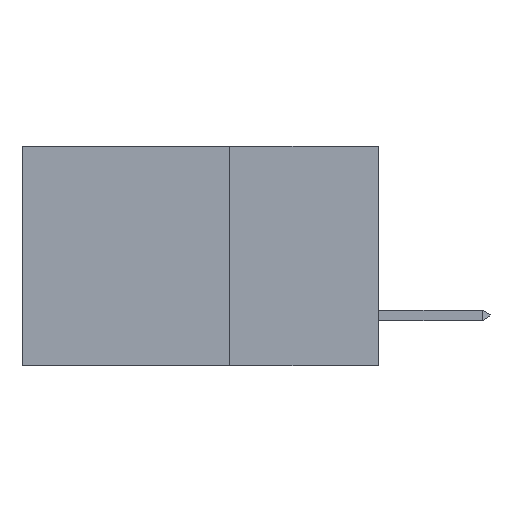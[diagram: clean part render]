
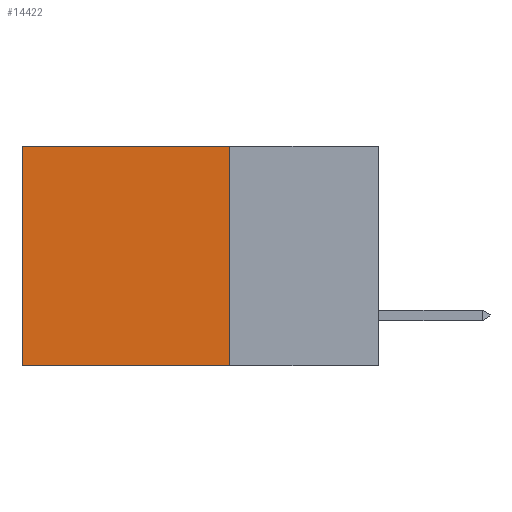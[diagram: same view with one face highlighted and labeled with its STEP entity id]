
A CAD part, left-side view. The second image highlights one B-rep face of the part: STEP entity #14422.
In plain terms, the highlighted planar face has unit normal (-1, 0, 0).
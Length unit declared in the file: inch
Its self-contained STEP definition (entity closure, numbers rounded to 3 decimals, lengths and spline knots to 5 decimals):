
#515 = CARTESIAN_POINT ( 'NONE',  ( 0.298, 0.25, 0. ) ) ;
#547 = CARTESIAN_POINT ( 'NONE',  ( 0.298, 0.6, 0. ) ) ;
#1889 = DIRECTION ( 'NONE',  ( 1., 0., 0. ) ) ;
#2542 = ORIENTED_EDGE ( 'NONE', *, *, #6276, .T. ) ;
#2660 = LINE ( 'NONE', #14740, #15370 ) ;
#3211 = EDGE_CURVE ( 'NONE', #7305, #8714, #5840, .T. ) ;
#3430 = EDGE_LOOP ( 'NONE', ( #2542, #12902, #21877, #7335 ) ) ;
#3825 = CARTESIAN_POINT ( 'NONE',  ( 0.298, 0.25, 0. ) ) ;
#4298 = LINE ( 'NONE', #515, #23408 ) ;
#5840 = LINE ( 'NONE', #8476, #15121 ) ;
#6066 = VERTEX_POINT ( 'NONE', #10850 ) ;
#6276 = EDGE_CURVE ( 'NONE', #6066, #8714, #20544, .T. ) ;
#6742 = EDGE_CURVE ( 'NONE', #23928, #6066, #4298, .T. ) ;
#6780 = DIRECTION ( 'NONE',  ( 0., 1., 0. ) ) ;
#7305 = VERTEX_POINT ( 'NONE', #9884 ) ;
#7335 = ORIENTED_EDGE ( 'NONE', *, *, #6742, .T. ) ;
#8476 = CARTESIAN_POINT ( 'NONE',  ( 0.298, 0.25, -0.37 ) ) ;
#8644 = VECTOR ( 'NONE', #15340, 39.37008 ) ;
#8714 = VERTEX_POINT ( 'NONE', #11927 ) ;
#9884 = CARTESIAN_POINT ( 'NONE',  ( 0.298, 0.25, -0.37 ) ) ;
#10850 = CARTESIAN_POINT ( 'NONE',  ( 0.298, 0.6, 0. ) ) ;
#11927 = CARTESIAN_POINT ( 'NONE',  ( 0.298, 0.6, -0.37 ) ) ;
#12902 = ORIENTED_EDGE ( 'NONE', *, *, #3211, .F. ) ;
#14422 = ADVANCED_FACE ( 'NONE', ( #17139 ), #22346, .F. ) ;
#14740 = CARTESIAN_POINT ( 'NONE',  ( 0.298, 0.25, 0. ) ) ;
#15048 = DIRECTION ( 'NONE',  ( 0., 0., -1. ) ) ;
#15121 = VECTOR ( 'NONE', #6780, 39.37008 ) ;
#15340 = DIRECTION ( 'NONE',  ( 0., 0., -1. ) ) ;
#15370 = VECTOR ( 'NONE', #16566, 39.37008 ) ;
#16566 = DIRECTION ( 'NONE',  ( 0., 0., -1. ) ) ;
#16973 = DIRECTION ( 'NONE',  ( 0., 1., 0. ) ) ;
#17139 = FACE_OUTER_BOUND ( 'NONE', #3430, .T. ) ;
#17673 = CARTESIAN_POINT ( 'NONE',  ( 0.298, 0.25, 0. ) ) ;
#17676 = AXIS2_PLACEMENT_3D ( 'NONE', #3825, #1889, #15048 ) ;
#20260 = EDGE_CURVE ( 'NONE', #23928, #7305, #2660, .T. ) ;
#20544 = LINE ( 'NONE', #547, #8644 ) ;
#21877 = ORIENTED_EDGE ( 'NONE', *, *, #20260, .F. ) ;
#22346 = PLANE ( 'NONE',  #17676 ) ;
#23408 = VECTOR ( 'NONE', #16973, 39.37008 ) ;
#23928 = VERTEX_POINT ( 'NONE', #17673 ) ;
